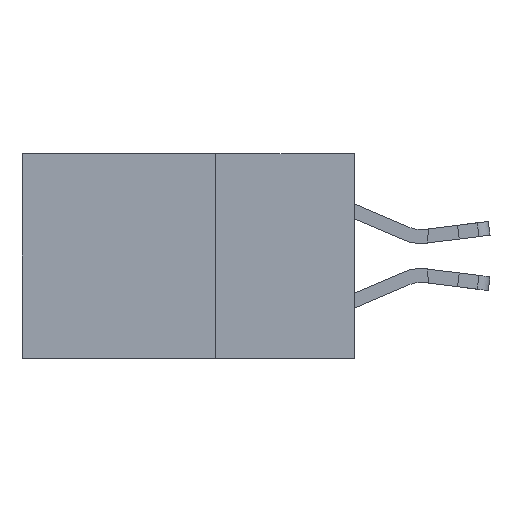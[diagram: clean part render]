
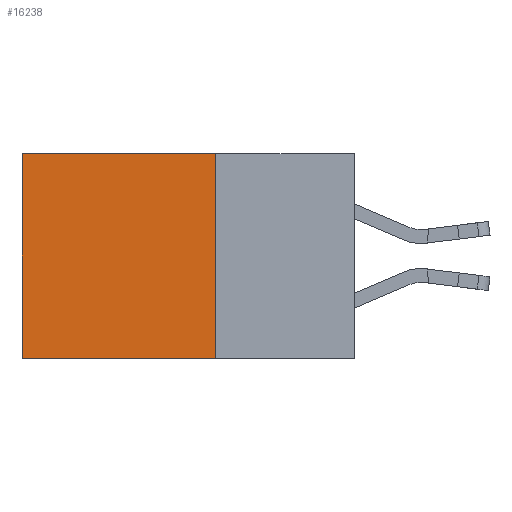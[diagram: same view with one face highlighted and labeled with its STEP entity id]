
A CAD part, left-side view. The second image highlights one B-rep face of the part: STEP entity #16238.
In plain terms, the highlighted planar face has unit normal (-1, 0, 0).
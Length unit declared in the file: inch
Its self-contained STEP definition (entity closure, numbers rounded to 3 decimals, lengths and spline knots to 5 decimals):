
#455 = VERTEX_POINT ( 'NONE', #6473 ) ;
#476 = DIRECTION ( 'NONE',  ( 0., 0., -1. ) ) ;
#522 = CARTESIAN_POINT ( 'NONE',  ( 0.298, 0.6, 0. ) ) ;
#1275 = DIRECTION ( 'NONE',  ( 1., 0., 0. ) ) ;
#1500 = LINE ( 'NONE', #7961, #9576 ) ;
#2092 = LINE ( 'NONE', #6165, #9726 ) ;
#2994 = CARTESIAN_POINT ( 'NONE',  ( 0.298, 0.25, 0. ) ) ;
#3250 = EDGE_CURVE ( 'NONE', #3284, #4546, #6251, .T. ) ;
#3284 = VERTEX_POINT ( 'NONE', #4255 ) ;
#3408 = VERTEX_POINT ( 'NONE', #17079 ) ;
#4142 = EDGE_LOOP ( 'NONE', ( #7274, #8800, #7885, #10371 ) ) ;
#4255 = CARTESIAN_POINT ( 'NONE',  ( 0.298, 0.25, 0. ) ) ;
#4546 = VERTEX_POINT ( 'NONE', #12103 ) ;
#5471 = CARTESIAN_POINT ( 'NONE',  ( 0.298, 0.25, 0. ) ) ;
#5791 = VECTOR ( 'NONE', #12258, 39.37008 ) ;
#6165 = CARTESIAN_POINT ( 'NONE',  ( 0.298, 0.25, -0.37 ) ) ;
#6251 = LINE ( 'NONE', #2994, #5791 ) ;
#6473 = CARTESIAN_POINT ( 'NONE',  ( 0.298, 0.6, 0. ) ) ;
#6539 = EDGE_CURVE ( 'NONE', #4546, #3408, #2092, .T. ) ;
#6775 = AXIS2_PLACEMENT_3D ( 'NONE', #5471, #1275, #11205 ) ;
#7274 = ORIENTED_EDGE ( 'NONE', *, *, #13564, .T. ) ;
#7800 = DIRECTION ( 'NONE',  ( 0., 1., 0. ) ) ;
#7885 = ORIENTED_EDGE ( 'NONE', *, *, #3250, .F. ) ;
#7961 = CARTESIAN_POINT ( 'NONE',  ( 0.298, 0.25, 0. ) ) ;
#8800 = ORIENTED_EDGE ( 'NONE', *, *, #6539, .F. ) ;
#9576 = VECTOR ( 'NONE', #7800, 39.37008 ) ;
#9726 = VECTOR ( 'NONE', #17114, 39.37008 ) ;
#9839 = PLANE ( 'NONE',  #6775 ) ;
#10371 = ORIENTED_EDGE ( 'NONE', *, *, #11265, .T. ) ;
#11205 = DIRECTION ( 'NONE',  ( 0., 0., -1. ) ) ;
#11265 = EDGE_CURVE ( 'NONE', #3284, #455, #1500, .T. ) ;
#11640 = LINE ( 'NONE', #522, #12086 ) ;
#12086 = VECTOR ( 'NONE', #476, 39.37008 ) ;
#12103 = CARTESIAN_POINT ( 'NONE',  ( 0.298, 0.25, -0.37 ) ) ;
#12258 = DIRECTION ( 'NONE',  ( 0., 0., -1. ) ) ;
#13564 = EDGE_CURVE ( 'NONE', #455, #3408, #11640, .T. ) ;
#15442 = FACE_OUTER_BOUND ( 'NONE', #4142, .T. ) ;
#16238 = ADVANCED_FACE ( 'NONE', ( #15442 ), #9839, .F. ) ;
#17079 = CARTESIAN_POINT ( 'NONE',  ( 0.298, 0.6, -0.37 ) ) ;
#17114 = DIRECTION ( 'NONE',  ( 0., 1., 0. ) ) ;
